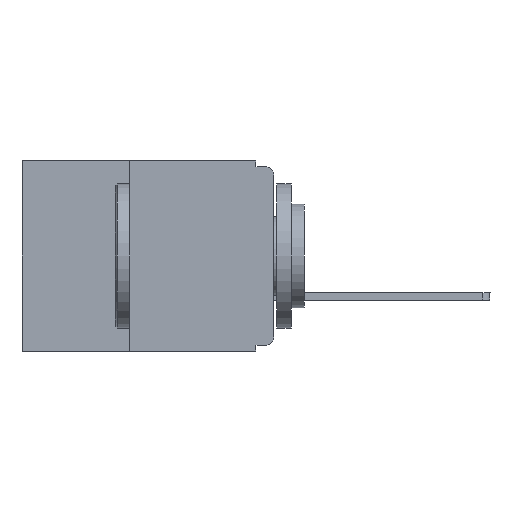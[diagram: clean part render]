
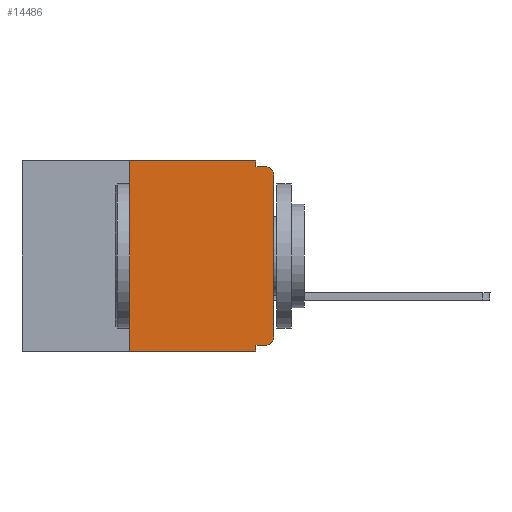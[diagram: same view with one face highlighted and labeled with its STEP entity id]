
A CAD part, left-side view. The second image highlights one B-rep face of the part: STEP entity #14486.
In plain terms, the highlighted planar face has unit normal (-1, 0, 0).
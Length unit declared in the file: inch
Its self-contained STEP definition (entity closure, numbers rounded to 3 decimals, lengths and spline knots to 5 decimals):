
#220 = LINE ( 'NONE', #5634, #6213 ) ;
#524 = CARTESIAN_POINT ( 'NONE',  ( 0., 0., -0.01 ) ) ;
#628 = VERTEX_POINT ( 'NONE', #10283 ) ;
#640 = EDGE_CURVE ( 'NONE', #13179, #1082, #12924, .T. ) ;
#701 = ORIENTED_EDGE ( 'NONE', *, *, #3488, .T. ) ;
#750 = CIRCLE ( 'NONE', #4684, 0.015 ) ;
#1082 = VERTEX_POINT ( 'NONE', #8077 ) ;
#1397 = CARTESIAN_POINT ( 'NONE',  ( 0., 0.015, -0.32 ) ) ;
#1926 = VERTEX_POINT ( 'NONE', #1397 ) ;
#2174 = VECTOR ( 'NONE', #14706, 39.37008 ) ;
#2330 = FACE_OUTER_BOUND ( 'NONE', #4342, .T. ) ;
#2423 = DIRECTION ( 'NONE',  ( 0., 0., 1. ) ) ;
#2981 = EDGE_CURVE ( 'NONE', #7728, #13179, #8556, .T. ) ;
#3012 = VERTEX_POINT ( 'NONE', #11649 ) ;
#3023 = CARTESIAN_POINT ( 'NONE',  ( 0., 0.015, -0.305 ) ) ;
#3114 = DIRECTION ( 'NONE',  ( -1., 0., 0. ) ) ;
#3177 = ORIENTED_EDGE ( 'NONE', *, *, #14380, .F. ) ;
#3488 = EDGE_CURVE ( 'NONE', #3012, #6695, #220, .T. ) ;
#3553 = CARTESIAN_POINT ( 'NONE',  ( 0., 0.031, -0.33 ) ) ;
#3580 = CARTESIAN_POINT ( 'NONE',  ( 0., 0.031, -0.32 ) ) ;
#3683 = CARTESIAN_POINT ( 'NONE',  ( 0., 0.437, -0.33 ) ) ;
#3808 = DIRECTION ( 'NONE',  ( 0., 0., -1. ) ) ;
#4090 = VECTOR ( 'NONE', #10113, 39.37008 ) ;
#4342 = EDGE_LOOP ( 'NONE', ( #701, #8809, #8022, #13868, #7035, #11889, #11412, #9332, #3177, #7725 ) ) ;
#4428 = CARTESIAN_POINT ( 'NONE',  ( 0., 0.031, 0. ) ) ;
#4523 = EDGE_CURVE ( 'NONE', #6695, #13431, #10059, .T. ) ;
#4641 = PLANE ( 'NONE',  #9609 ) ;
#4684 = AXIS2_PLACEMENT_3D ( 'NONE', #3023, #5329, #5438 ) ;
#4690 = DIRECTION ( 'NONE',  ( 1., 0., 0. ) ) ;
#4831 = LINE ( 'NONE', #6846, #13577 ) ;
#4872 = VECTOR ( 'NONE', #5530, 39.37008 ) ;
#5329 = DIRECTION ( 'NONE',  ( -1., 0., 0. ) ) ;
#5438 = DIRECTION ( 'NONE',  ( 0., 0., -1. ) ) ;
#5530 = DIRECTION ( 'NONE',  ( 0., -1., 0. ) ) ;
#5634 = CARTESIAN_POINT ( 'NONE',  ( 0., 0., 0. ) ) ;
#5937 = EDGE_CURVE ( 'NONE', #15677, #13859, #12749, .T. ) ;
#6169 = VECTOR ( 'NONE', #2423, 39.37008 ) ;
#6213 = VECTOR ( 'NONE', #14459, 39.37008 ) ;
#6695 = VERTEX_POINT ( 'NONE', #9589 ) ;
#6846 = CARTESIAN_POINT ( 'NONE',  ( 0., 0., -0.32 ) ) ;
#7035 = ORIENTED_EDGE ( 'NONE', *, *, #2981, .F. ) ;
#7125 = DIRECTION ( 'NONE',  ( 0., 0., -1. ) ) ;
#7571 = LINE ( 'NONE', #3683, #2174 ) ;
#7603 = EDGE_CURVE ( 'NONE', #1082, #13431, #15556, .T. ) ;
#7725 = ORIENTED_EDGE ( 'NONE', *, *, #10745, .T. ) ;
#7728 = VERTEX_POINT ( 'NONE', #14463 ) ;
#8022 = ORIENTED_EDGE ( 'NONE', *, *, #7603, .F. ) ;
#8077 = CARTESIAN_POINT ( 'NONE',  ( 0., 0.031, -0.01 ) ) ;
#8543 = CARTESIAN_POINT ( 'NONE',  ( 0., 0.015, -0.01 ) ) ;
#8556 = LINE ( 'NONE', #12511, #4090 ) ;
#8781 = EDGE_CURVE ( 'NONE', #628, #13859, #7571, .T. ) ;
#8797 = VECTOR ( 'NONE', #7125, 39.37008 ) ;
#8809 = ORIENTED_EDGE ( 'NONE', *, *, #4523, .T. ) ;
#9073 = AXIS2_PLACEMENT_3D ( 'NONE', #10534, #3114, #9317 ) ;
#9317 = DIRECTION ( 'NONE',  ( 0., 0., -1. ) ) ;
#9332 = ORIENTED_EDGE ( 'NONE', *, *, #5937, .F. ) ;
#9589 = CARTESIAN_POINT ( 'NONE',  ( 0., 0., -0.025 ) ) ;
#9609 = AXIS2_PLACEMENT_3D ( 'NONE', #12079, #4690, #13335 ) ;
#10059 = CIRCLE ( 'NONE', #9073, 0.015 ) ;
#10113 = DIRECTION ( 'NONE',  ( 0., -1., 0. ) ) ;
#10283 = CARTESIAN_POINT ( 'NONE',  ( 0., 0.25, -0.33 ) ) ;
#10534 = CARTESIAN_POINT ( 'NONE',  ( 0., 0.015, -0.025 ) ) ;
#10745 = EDGE_CURVE ( 'NONE', #1926, #3012, #750, .T. ) ;
#11412 = ORIENTED_EDGE ( 'NONE', *, *, #8781, .T. ) ;
#11649 = CARTESIAN_POINT ( 'NONE',  ( 0., 0., -0.305 ) ) ;
#11889 = ORIENTED_EDGE ( 'NONE', *, *, #14676, .F. ) ;
#11960 = VECTOR ( 'NONE', #3808, 39.37008 ) ;
#12079 = CARTESIAN_POINT ( 'NONE',  ( 0., 0.437, 0. ) ) ;
#12400 = LINE ( 'NONE', #15000, #6169 ) ;
#12511 = CARTESIAN_POINT ( 'NONE',  ( 0., 0.437, 0. ) ) ;
#12749 = LINE ( 'NONE', #14997, #11960 ) ;
#12924 = LINE ( 'NONE', #14040, #8797 ) ;
#13179 = VERTEX_POINT ( 'NONE', #4428 ) ;
#13335 = DIRECTION ( 'NONE',  ( 0., 0., -1. ) ) ;
#13431 = VERTEX_POINT ( 'NONE', #8543 ) ;
#13577 = VECTOR ( 'NONE', #15550, 39.37008 ) ;
#13859 = VERTEX_POINT ( 'NONE', #3553 ) ;
#13868 = ORIENTED_EDGE ( 'NONE', *, *, #640, .F. ) ;
#14040 = CARTESIAN_POINT ( 'NONE',  ( 0., 0.031, 0. ) ) ;
#14380 = EDGE_CURVE ( 'NONE', #1926, #15677, #4831, .T. ) ;
#14459 = DIRECTION ( 'NONE',  ( 0., 0., 1. ) ) ;
#14463 = CARTESIAN_POINT ( 'NONE',  ( 0., 0.25, 0. ) ) ;
#14486 = ADVANCED_FACE ( 'NONE', ( #2330 ), #4641, .F. ) ;
#14676 = EDGE_CURVE ( 'NONE', #628, #7728, #12400, .T. ) ;
#14706 = DIRECTION ( 'NONE',  ( 0., -1., 0. ) ) ;
#14997 = CARTESIAN_POINT ( 'NONE',  ( 0., 0.031, -0.33 ) ) ;
#15000 = CARTESIAN_POINT ( 'NONE',  ( 0., 0.25, -0.33 ) ) ;
#15550 = DIRECTION ( 'NONE',  ( 0., 1., 0. ) ) ;
#15556 = LINE ( 'NONE', #524, #4872 ) ;
#15677 = VERTEX_POINT ( 'NONE', #3580 ) ;
